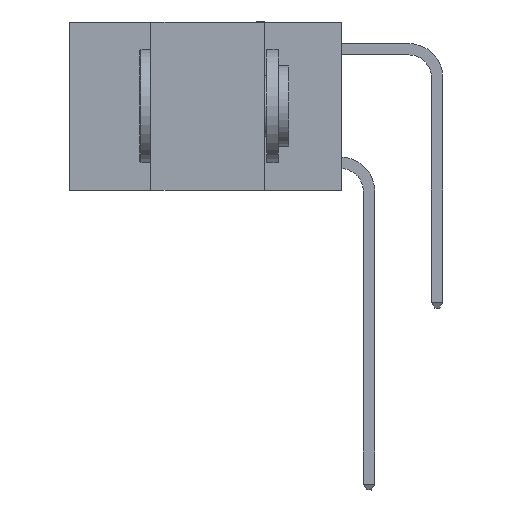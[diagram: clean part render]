
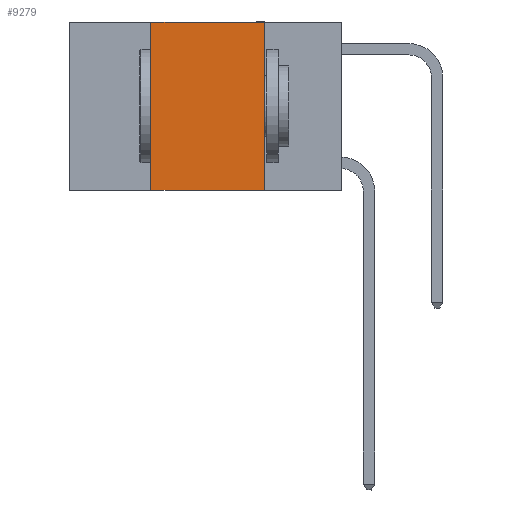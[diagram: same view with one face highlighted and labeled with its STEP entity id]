
A CAD part, left-side view. The second image highlights one B-rep face of the part: STEP entity #9279.
In plain terms, the highlighted planar face has unit normal (-1, 0, 0).
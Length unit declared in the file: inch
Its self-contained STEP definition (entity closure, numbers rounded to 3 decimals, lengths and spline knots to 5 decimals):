
#256 = AXIS2_PLACEMENT_3D ( 'NONE', #16939, #25838, #5826 ) ;
#1165 = ORIENTED_EDGE ( 'NONE', *, *, #20198, .F. ) ;
#1708 = VECTOR ( 'NONE', #12987, 39.37008 ) ;
#3899 = CARTESIAN_POINT ( 'NONE',  ( 0., 0.42, 0. ) ) ;
#3948 = CARTESIAN_POINT ( 'NONE',  ( 0., 0.17, -0.37 ) ) ;
#3994 = VERTEX_POINT ( 'NONE', #3948 ) ;
#5718 = EDGE_CURVE ( 'NONE', #23329, #3994, #10501, .T. ) ;
#5826 = DIRECTION ( 'NONE',  ( 0., 0., -1. ) ) ;
#6270 = CARTESIAN_POINT ( 'NONE',  ( 0., 0.6, -0.37 ) ) ;
#8041 = PLANE ( 'NONE',  #256 ) ;
#8297 = CARTESIAN_POINT ( 'NONE',  ( 0., 0.42, -0.37 ) ) ;
#8692 = DIRECTION ( 'NONE',  ( 0., 0., 1. ) ) ;
#9044 = CARTESIAN_POINT ( 'NONE',  ( 0., 0.6, 0. ) ) ;
#9279 = ADVANCED_FACE ( 'NONE', ( #28038 ), #8041, .F. ) ;
#10501 = LINE ( 'NONE', #6270, #24971 ) ;
#11822 = EDGE_CURVE ( 'NONE', #19634, #3994, #21232, .T. ) ;
#12872 = EDGE_LOOP ( 'NONE', ( #14419, #1165, #17572, #21239 ) ) ;
#12987 = DIRECTION ( 'NONE',  ( 0., -1., 0. ) ) ;
#13282 = LINE ( 'NONE', #9044, #1708 ) ;
#14419 = ORIENTED_EDGE ( 'NONE', *, *, #11822, .F. ) ;
#14874 = VECTOR ( 'NONE', #8692, 39.37008 ) ;
#16312 = EDGE_CURVE ( 'NONE', #23329, #25469, #24330, .T. ) ;
#16695 = VECTOR ( 'NONE', #27800, 39.37008 ) ;
#16939 = CARTESIAN_POINT ( 'NONE',  ( 0., 0.6, 0. ) ) ;
#17572 = ORIENTED_EDGE ( 'NONE', *, *, #16312, .F. ) ;
#19323 = CARTESIAN_POINT ( 'NONE',  ( 0., 0.17, 0. ) ) ;
#19634 = VERTEX_POINT ( 'NONE', #19323 ) ;
#19857 = DIRECTION ( 'NONE',  ( 0., -1., 0. ) ) ;
#20198 = EDGE_CURVE ( 'NONE', #25469, #19634, #13282, .T. ) ;
#20672 = CARTESIAN_POINT ( 'NONE',  ( 0., 0.17, 0. ) ) ;
#21232 = LINE ( 'NONE', #20672, #16695 ) ;
#21239 = ORIENTED_EDGE ( 'NONE', *, *, #5718, .T. ) ;
#23329 = VERTEX_POINT ( 'NONE', #8297 ) ;
#24330 = LINE ( 'NONE', #28699, #14874 ) ;
#24971 = VECTOR ( 'NONE', #19857, 39.37008 ) ;
#25469 = VERTEX_POINT ( 'NONE', #3899 ) ;
#25838 = DIRECTION ( 'NONE',  ( 1., 0., 0. ) ) ;
#27800 = DIRECTION ( 'NONE',  ( 0., 0., -1. ) ) ;
#28038 = FACE_OUTER_BOUND ( 'NONE', #12872, .T. ) ;
#28699 = CARTESIAN_POINT ( 'NONE',  ( 0., 0.42, 0. ) ) ;
